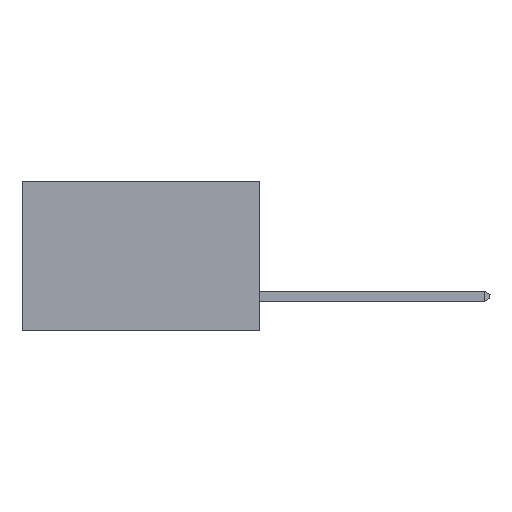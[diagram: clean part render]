
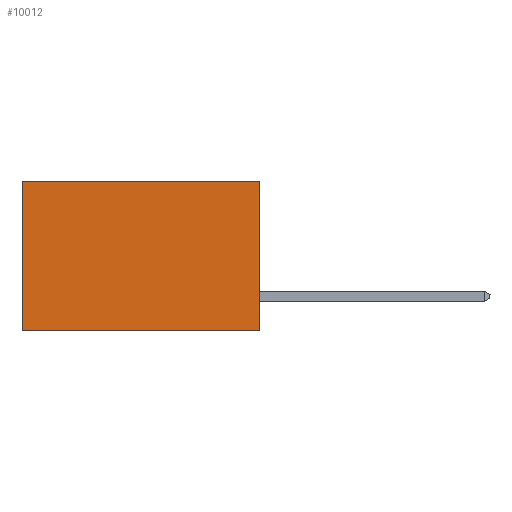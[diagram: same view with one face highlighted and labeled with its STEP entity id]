
A CAD part, left-side view. The second image highlights one B-rep face of the part: STEP entity #10012.
In plain terms, the highlighted planar face has unit normal (-1, 0, 0).
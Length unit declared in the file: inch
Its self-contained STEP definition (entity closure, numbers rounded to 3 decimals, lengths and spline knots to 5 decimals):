
#922 = VECTOR ( 'NONE', #4868, 39.37008 ) ;
#1178 = LINE ( 'NONE', #1612, #11366 ) ;
#1295 = VECTOR ( 'NONE', #5311, 39.37008 ) ;
#1404 = ORIENTED_EDGE ( 'NONE', *, *, #7336, .T. ) ;
#1612 = CARTESIAN_POINT ( 'NONE',  ( 0.277, 0., -0.37 ) ) ;
#2187 = CARTESIAN_POINT ( 'NONE',  ( 0.277, 0., 0. ) ) ;
#2356 = CARTESIAN_POINT ( 'NONE',  ( 0.277, 0., -0.37 ) ) ;
#2365 = LINE ( 'NONE', #12053, #7357 ) ;
#2926 = VERTEX_POINT ( 'NONE', #2187 ) ;
#3091 = DIRECTION ( 'NONE',  ( 0., 1., 0. ) ) ;
#3913 = LINE ( 'NONE', #5457, #1295 ) ;
#4322 = CARTESIAN_POINT ( 'NONE',  ( 0.277, 0., -0.37 ) ) ;
#4396 = VERTEX_POINT ( 'NONE', #10198 ) ;
#4868 = DIRECTION ( 'NONE',  ( 0., 0., -1. ) ) ;
#4993 = EDGE_LOOP ( 'NONE', ( #1404, #11680, #12211, #8706 ) ) ;
#5311 = DIRECTION ( 'NONE',  ( 0., 0., -1. ) ) ;
#5336 = DIRECTION ( 'NONE',  ( 1., 0., 0. ) ) ;
#5457 = CARTESIAN_POINT ( 'NONE',  ( 0.277, 0.59, -0.37 ) ) ;
#5730 = CARTESIAN_POINT ( 'NONE',  ( 0.277, 0., -0.37 ) ) ;
#6004 = EDGE_CURVE ( 'NONE', #6032, #6939, #1178, .T. ) ;
#6032 = VERTEX_POINT ( 'NONE', #2356 ) ;
#6939 = VERTEX_POINT ( 'NONE', #10399 ) ;
#7336 = EDGE_CURVE ( 'NONE', #4396, #6939, #3913, .T. ) ;
#7357 = VECTOR ( 'NONE', #12619, 39.37008 ) ;
#7925 = EDGE_CURVE ( 'NONE', #2926, #6032, #11163, .T. ) ;
#7984 = EDGE_CURVE ( 'NONE', #2926, #4396, #2365, .T. ) ;
#8706 = ORIENTED_EDGE ( 'NONE', *, *, #7984, .T. ) ;
#10012 = ADVANCED_FACE ( 'NONE', ( #11305 ), #10278, .F. ) ;
#10198 = CARTESIAN_POINT ( 'NONE',  ( 0.277, 0.59, 0. ) ) ;
#10278 = PLANE ( 'NONE',  #11050 ) ;
#10399 = CARTESIAN_POINT ( 'NONE',  ( 0.277, 0.59, -0.37 ) ) ;
#11050 = AXIS2_PLACEMENT_3D ( 'NONE', #4322, #5336, #12075 ) ;
#11163 = LINE ( 'NONE', #5730, #922 ) ;
#11305 = FACE_OUTER_BOUND ( 'NONE', #4993, .T. ) ;
#11366 = VECTOR ( 'NONE', #3091, 39.37008 ) ;
#11680 = ORIENTED_EDGE ( 'NONE', *, *, #6004, .F. ) ;
#12053 = CARTESIAN_POINT ( 'NONE',  ( 0.277, 0., 0. ) ) ;
#12075 = DIRECTION ( 'NONE',  ( 0., 0., -1. ) ) ;
#12211 = ORIENTED_EDGE ( 'NONE', *, *, #7925, .F. ) ;
#12619 = DIRECTION ( 'NONE',  ( 0., 1., 0. ) ) ;
